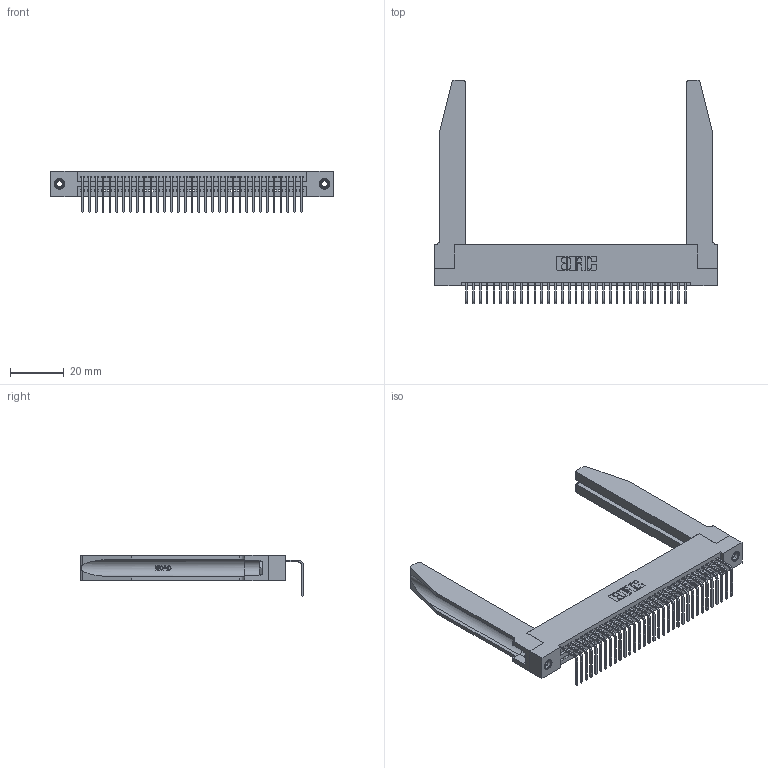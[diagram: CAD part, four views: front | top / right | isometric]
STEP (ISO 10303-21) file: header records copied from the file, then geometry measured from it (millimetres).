
FILE_DESCRIPTION (( 'STEP AP203' ), '1' );
FILE_NAME ('345-033-558-178.STEP', '2019-10-10T14:44:31', ( '' ), ( '' ), 'SwSTEP 2.0', 'SolidWorks 2016', '' );
FILE_SCHEMA (( 'CONFIG_CONTROL_DESIGN' ));
Length unit declared in the file: inch
Products named in the file (5): 345 Part_Flush Mounting Lugs - 0.156 Dia-TH; 345-292-001_558 Tail - 2; 345-250-001_345-250-001-102; 345-220-078_345-220-078; 345-033-558-178
Assembly tree (38 placements, depth 2):
  345-033-558-178
    345 Part_Flush Mounting Lugs - 0.156 Dia-TH
    345-292-001_558 Tail - 2  x33
    345-250-001_345-250-001-102  x2
    345-220-078_345-220-078  x2
Bounding box: 105.05 x 82.79 x 15.37 mm (x, y, z)
Volume: 17784.9 mm3; surface area: 20677.6 mm2
Topology: 38 solids, 38 shells, 2340 faces, 6955 edges, 4582 vertices
Faces by surface type: plane 1608, cylinder 680, bspline 36, cone 12, torus 4
Entity records: 30872 total; most frequent: CARTESIAN_POINT 6246, ORIENTED_EDGE 5110, DIRECTION 4475, EDGE_CURVE 2555, LINE 2197, VECTOR 2197, VERTEX_POINT 1696, AXIS2_PLACEMENT_3D 1139
